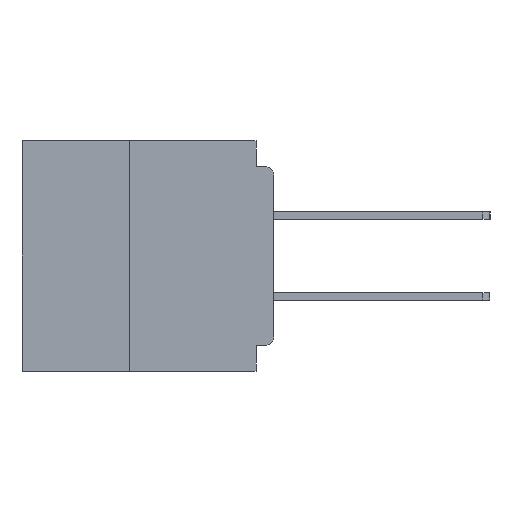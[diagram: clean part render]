
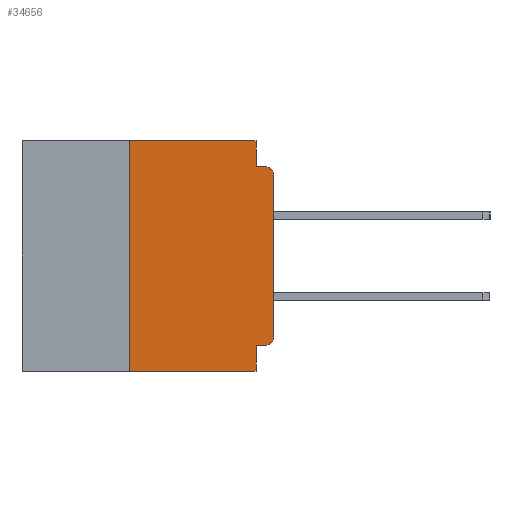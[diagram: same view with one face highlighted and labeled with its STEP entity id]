
A CAD part, left-side view. The second image highlights one B-rep face of the part: STEP entity #34656.
In plain terms, the highlighted planar face has unit normal (-1, 0, 0).
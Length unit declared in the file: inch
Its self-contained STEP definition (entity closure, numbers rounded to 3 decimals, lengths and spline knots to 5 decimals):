
#168 = LINE ( 'NONE', #18162, #8839 ) ;
#346 = CARTESIAN_POINT ( 'NONE',  ( 0., 0.031, -0.4 ) ) ;
#747 = VERTEX_POINT ( 'NONE', #43835 ) ;
#914 = CARTESIAN_POINT ( 'NONE',  ( 0., 0.015, -0.34 ) ) ;
#1151 = DIRECTION ( 'NONE',  ( -1., 0., 0. ) ) ;
#1240 = EDGE_CURVE ( 'NONE', #22792, #47048, #10322, .T. ) ;
#1352 = DIRECTION ( 'NONE',  ( 0., 1., 0. ) ) ;
#1519 = ORIENTED_EDGE ( 'NONE', *, *, #35724, .F. ) ;
#1993 = CARTESIAN_POINT ( 'NONE',  ( 0., 0.25, -0.4 ) ) ;
#2025 = VECTOR ( 'NONE', #4063, 39.37008 ) ;
#2421 = PLANE ( 'NONE',  #27159 ) ;
#2476 = CARTESIAN_POINT ( 'NONE',  ( 0., 0., -0.06 ) ) ;
#4063 = DIRECTION ( 'NONE',  ( 0., 0., -1. ) ) ;
#4639 = DIRECTION ( 'NONE',  ( 0., 0., -1. ) ) ;
#5277 = VECTOR ( 'NONE', #39889, 39.37008 ) ;
#5843 = DIRECTION ( 'NONE',  ( 0., 0., 1. ) ) ;
#6106 = CARTESIAN_POINT ( 'NONE',  ( 0., 0.437, 0. ) ) ;
#7313 = VERTEX_POINT ( 'NONE', #2476 ) ;
#8318 = VECTOR ( 'NONE', #22296, 39.37008 ) ;
#8490 = CARTESIAN_POINT ( 'NONE',  ( 0., 0.015, -0.045 ) ) ;
#8497 = FACE_OUTER_BOUND ( 'NONE', #19519, .T. ) ;
#8839 = VECTOR ( 'NONE', #10776, 39.37008 ) ;
#8974 = VECTOR ( 'NONE', #15492, 39.37008 ) ;
#9114 = ORIENTED_EDGE ( 'NONE', *, *, #36765, .T. ) ;
#9721 = ORIENTED_EDGE ( 'NONE', *, *, #42004, .F. ) ;
#9819 = DIRECTION ( 'NONE',  ( 1., 0., 0. ) ) ;
#10322 = LINE ( 'NONE', #24551, #20125 ) ;
#10776 = DIRECTION ( 'NONE',  ( 0., -1., 0. ) ) ;
#10883 = ORIENTED_EDGE ( 'NONE', *, *, #22051, .T. ) ;
#12954 = LINE ( 'NONE', #346, #2025 ) ;
#13799 = EDGE_CURVE ( 'NONE', #31691, #747, #168, .T. ) ;
#14006 = LINE ( 'NONE', #16906, #31336 ) ;
#14074 = CARTESIAN_POINT ( 'NONE',  ( 0., 0.25, -0.4 ) ) ;
#14693 = VECTOR ( 'NONE', #23814, 39.37008 ) ;
#15492 = DIRECTION ( 'NONE',  ( 0., -1., 0. ) ) ;
#16906 = CARTESIAN_POINT ( 'NONE',  ( 0., 0., 0. ) ) ;
#16911 = CARTESIAN_POINT ( 'NONE',  ( 0., 0.015, -0.355 ) ) ;
#18162 = CARTESIAN_POINT ( 'NONE',  ( 0., 0.437, 0. ) ) ;
#18599 = CARTESIAN_POINT ( 'NONE',  ( 0., 0.437, -0.4 ) ) ;
#19519 = EDGE_LOOP ( 'NONE', ( #9114, #19976, #1519, #23155, #32030, #31985, #33666, #9721, #38772, #10883 ) ) ;
#19976 = ORIENTED_EDGE ( 'NONE', *, *, #42115, .T. ) ;
#20125 = VECTOR ( 'NONE', #1352, 39.37008 ) ;
#20453 = CARTESIAN_POINT ( 'NONE',  ( 0., 0.031, -0.4 ) ) ;
#22051 = EDGE_CURVE ( 'NONE', #22792, #27639, #33627, .T. ) ;
#22296 = DIRECTION ( 'NONE',  ( 0., -1., 0. ) ) ;
#22757 = VERTEX_POINT ( 'NONE', #1993 ) ;
#22792 = VERTEX_POINT ( 'NONE', #16911 ) ;
#23155 = ORIENTED_EDGE ( 'NONE', *, *, #31869, .F. ) ;
#23202 = CARTESIAN_POINT ( 'NONE',  ( 0., 0.015, -0.06 ) ) ;
#23814 = DIRECTION ( 'NONE',  ( 0., 0., -1. ) ) ;
#24551 = CARTESIAN_POINT ( 'NONE',  ( 0., 0., -0.355 ) ) ;
#25632 = CIRCLE ( 'NONE', #41030, 0.015 ) ;
#26493 = CARTESIAN_POINT ( 'NONE',  ( 0., 0., -0.045 ) ) ;
#26700 = DIRECTION ( 'NONE',  ( -1., 0., 0. ) ) ;
#26926 = DIRECTION ( 'NONE',  ( 0., 0., -1. ) ) ;
#27159 = AXIS2_PLACEMENT_3D ( 'NONE', #6106, #9819, #35589 ) ;
#27639 = VERTEX_POINT ( 'NONE', #37617 ) ;
#28897 = VERTEX_POINT ( 'NONE', #8490 ) ;
#31235 = CARTESIAN_POINT ( 'NONE',  ( 0., 0.031, 0. ) ) ;
#31336 = VECTOR ( 'NONE', #5843, 39.37008 ) ;
#31691 = VERTEX_POINT ( 'NONE', #44861 ) ;
#31869 = EDGE_CURVE ( 'NONE', #747, #40559, #33156, .T. ) ;
#31985 = ORIENTED_EDGE ( 'NONE', *, *, #44840, .F. ) ;
#32030 = ORIENTED_EDGE ( 'NONE', *, *, #13799, .F. ) ;
#32164 = CARTESIAN_POINT ( 'NONE',  ( 0., 0.031, -0.045 ) ) ;
#33156 = LINE ( 'NONE', #31235, #14693 ) ;
#33627 = CIRCLE ( 'NONE', #39297, 0.015 ) ;
#33666 = ORIENTED_EDGE ( 'NONE', *, *, #36416, .T. ) ;
#34656 = ADVANCED_FACE ( 'NONE', ( #8497 ), #2421, .F. ) ;
#34724 = CARTESIAN_POINT ( 'NONE',  ( 0., 0.031, -0.355 ) ) ;
#35589 = DIRECTION ( 'NONE',  ( 0., 0., -1. ) ) ;
#35724 = EDGE_CURVE ( 'NONE', #40559, #28897, #38378, .T. ) ;
#36416 = EDGE_CURVE ( 'NONE', #22757, #42312, #37735, .T. ) ;
#36765 = EDGE_CURVE ( 'NONE', #27639, #7313, #14006, .T. ) ;
#37617 = CARTESIAN_POINT ( 'NONE',  ( 0., 0., -0.34 ) ) ;
#37735 = LINE ( 'NONE', #18599, #8318 ) ;
#38378 = LINE ( 'NONE', #26493, #8974 ) ;
#38772 = ORIENTED_EDGE ( 'NONE', *, *, #1240, .F. ) ;
#39297 = AXIS2_PLACEMENT_3D ( 'NONE', #914, #26700, #4639 ) ;
#39889 = DIRECTION ( 'NONE',  ( 0., 0., 1. ) ) ;
#40559 = VERTEX_POINT ( 'NONE', #32164 ) ;
#40972 = LINE ( 'NONE', #14074, #5277 ) ;
#41030 = AXIS2_PLACEMENT_3D ( 'NONE', #23202, #1151, #26926 ) ;
#42004 = EDGE_CURVE ( 'NONE', #47048, #42312, #12954, .T. ) ;
#42115 = EDGE_CURVE ( 'NONE', #7313, #28897, #25632, .T. ) ;
#42312 = VERTEX_POINT ( 'NONE', #20453 ) ;
#43835 = CARTESIAN_POINT ( 'NONE',  ( 0., 0.031, 0. ) ) ;
#44840 = EDGE_CURVE ( 'NONE', #22757, #31691, #40972, .T. ) ;
#44861 = CARTESIAN_POINT ( 'NONE',  ( 0., 0.25, 0. ) ) ;
#47048 = VERTEX_POINT ( 'NONE', #34724 ) ;
